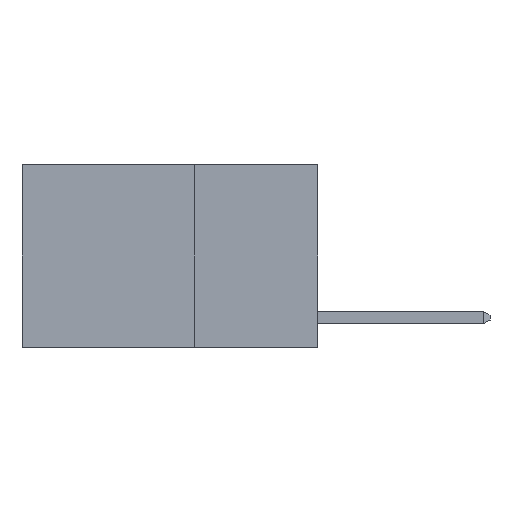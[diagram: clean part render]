
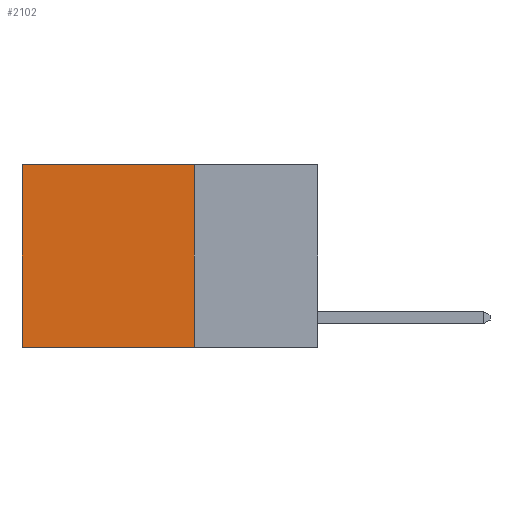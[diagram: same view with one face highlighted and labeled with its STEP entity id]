
A CAD part, left-side view. The second image highlights one B-rep face of the part: STEP entity #2102.
In plain terms, the highlighted planar face has unit normal (-1, 0, 0).
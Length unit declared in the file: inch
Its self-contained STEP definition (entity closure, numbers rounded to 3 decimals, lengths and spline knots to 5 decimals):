
#28 = VERTEX_POINT ( 'NONE', #8870 ) ;
#657 = EDGE_CURVE ( 'NONE', #3083, #6759, #3986, .T. ) ;
#717 = EDGE_LOOP ( 'NONE', ( #1714, #1719, #1752, #1761 ) ) ;
#1714 = ORIENTED_EDGE ( 'NONE', *, *, #6294, .T. ) ;
#1719 = ORIENTED_EDGE ( 'NONE', *, *, #9548, .F. ) ;
#1752 = ORIENTED_EDGE ( 'NONE', *, *, #7628, .F. ) ;
#1761 = ORIENTED_EDGE ( 'NONE', *, *, #657, .T. ) ;
#1941 = CARTESIAN_POINT ( 'NONE',  ( 0.2625, 0.6, 0. ) ) ;
#2102 = ADVANCED_FACE ( 'NONE', ( #5600 ), #6999, .F. ) ;
#3075 = VECTOR ( 'NONE', #3380, 39.37008 ) ;
#3083 = VERTEX_POINT ( 'NONE', #5902 ) ;
#3211 = CARTESIAN_POINT ( 'NONE',  ( 0.2625, 0.25, 0. ) ) ;
#3228 = DIRECTION ( 'NONE',  ( 0., 1., 0. ) ) ;
#3380 = DIRECTION ( 'NONE',  ( 0., 0., -1. ) ) ;
#3986 = LINE ( 'NONE', #3211, #7499 ) ;
#4694 = CARTESIAN_POINT ( 'NONE',  ( 0.2625, 0.25, -0.37 ) ) ;
#5325 = VECTOR ( 'NONE', #7787, 39.37008 ) ;
#5600 = FACE_OUTER_BOUND ( 'NONE', #717, .T. ) ;
#5772 = LINE ( 'NONE', #7114, #5325 ) ;
#5902 = CARTESIAN_POINT ( 'NONE',  ( 0.2625, 0.25, 0. ) ) ;
#6089 = VERTEX_POINT ( 'NONE', #6123 ) ;
#6123 = CARTESIAN_POINT ( 'NONE',  ( 0.2625, 0.6, -0.37 ) ) ;
#6294 = EDGE_CURVE ( 'NONE', #6759, #6089, #6950, .T. ) ;
#6300 = VECTOR ( 'NONE', #3228, 39.37008 ) ;
#6759 = VERTEX_POINT ( 'NONE', #1941 ) ;
#6920 = DIRECTION ( 'NONE',  ( 0., 0., -1. ) ) ;
#6950 = LINE ( 'NONE', #7619, #3075 ) ;
#6970 = DIRECTION ( 'NONE',  ( 1., 0., 0. ) ) ;
#6994 = CARTESIAN_POINT ( 'NONE',  ( 0.2625, 0.25, 0. ) ) ;
#6999 = PLANE ( 'NONE',  #7681 ) ;
#7114 = CARTESIAN_POINT ( 'NONE',  ( 0.2625, 0.25, 0. ) ) ;
#7499 = VECTOR ( 'NONE', #8811, 39.37008 ) ;
#7619 = CARTESIAN_POINT ( 'NONE',  ( 0.2625, 0.6, 0. ) ) ;
#7628 = EDGE_CURVE ( 'NONE', #3083, #28, #5772, .T. ) ;
#7681 = AXIS2_PLACEMENT_3D ( 'NONE', #6994, #6970, #6920 ) ;
#7787 = DIRECTION ( 'NONE',  ( 0., 0., -1. ) ) ;
#8076 = LINE ( 'NONE', #4694, #6300 ) ;
#8811 = DIRECTION ( 'NONE',  ( 0., 1., 0. ) ) ;
#8870 = CARTESIAN_POINT ( 'NONE',  ( 0.2625, 0.25, -0.37 ) ) ;
#9548 = EDGE_CURVE ( 'NONE', #28, #6089, #8076, .T. ) ;
